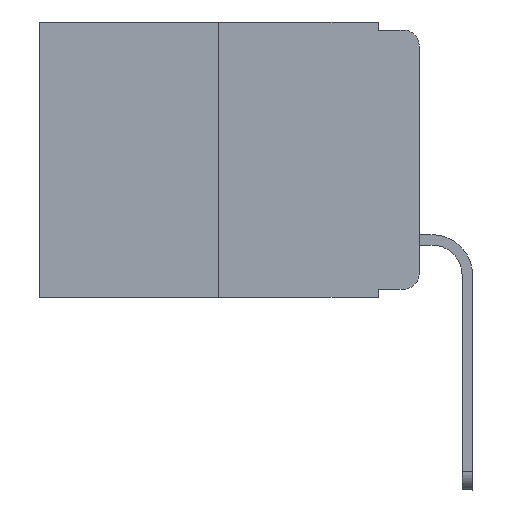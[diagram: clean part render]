
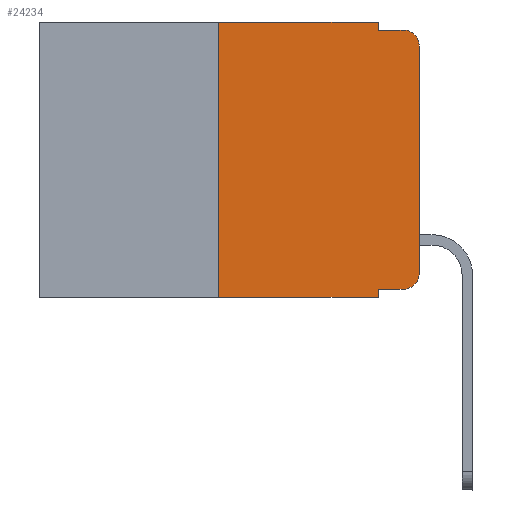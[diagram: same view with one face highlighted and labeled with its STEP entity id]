
A CAD part, left-side view. The second image highlights one B-rep face of the part: STEP entity #24234.
In plain terms, the highlighted planar face has unit normal (-1, 0, 0).
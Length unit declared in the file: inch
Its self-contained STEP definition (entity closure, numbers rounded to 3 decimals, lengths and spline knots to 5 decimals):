
#444 = DIRECTION ( 'NONE',  ( -1., 0., 0. ) ) ;
#1113 = VECTOR ( 'NONE', #25519, 39.37008 ) ;
#1357 = CARTESIAN_POINT ( 'NONE',  ( 0., 0., -0.313 ) ) ;
#1689 = VECTOR ( 'NONE', #13543, 39.37008 ) ;
#2533 = DIRECTION ( 'NONE',  ( 0., 0., -1. ) ) ;
#2951 = AXIS2_PLACEMENT_3D ( 'NONE', #6365, #25494, #16071 ) ;
#3312 = VERTEX_POINT ( 'NONE', #7951 ) ;
#3314 = EDGE_CURVE ( 'NONE', #19321, #23801, #14136, .T. ) ;
#3338 = PLANE ( 'NONE',  #13207 ) ;
#3358 = ORIENTED_EDGE ( 'NONE', *, *, #18865, .T. ) ;
#3513 = ORIENTED_EDGE ( 'NONE', *, *, #6354, .F. ) ;
#3849 = VERTEX_POINT ( 'NONE', #24023 ) ;
#4046 = LINE ( 'NONE', #19809, #18910 ) ;
#4088 = ORIENTED_EDGE ( 'NONE', *, *, #21610, .T. ) ;
#4286 = CARTESIAN_POINT ( 'NONE',  ( 0., 0., -0.03 ) ) ;
#4372 = EDGE_CURVE ( 'NONE', #3312, #18148, #19312, .T. ) ;
#4451 = VERTEX_POINT ( 'NONE', #1357 ) ;
#4537 = CARTESIAN_POINT ( 'NONE',  ( 0., 0.473, 0. ) ) ;
#5300 = DIRECTION ( 'NONE',  ( 1., 0., 0. ) ) ;
#5355 = CARTESIAN_POINT ( 'NONE',  ( 0., 0.051, -0.333 ) ) ;
#5700 = ORIENTED_EDGE ( 'NONE', *, *, #12153, .F. ) ;
#6138 = CARTESIAN_POINT ( 'NONE',  ( 0., 0.051, -0.01 ) ) ;
#6354 = EDGE_CURVE ( 'NONE', #18148, #3849, #22216, .T. ) ;
#6365 = CARTESIAN_POINT ( 'NONE',  ( 0., 0.02, -0.03 ) ) ;
#7677 = DIRECTION ( 'NONE',  ( 0., -1., 0. ) ) ;
#7944 = LINE ( 'NONE', #23806, #9525 ) ;
#7951 = CARTESIAN_POINT ( 'NONE',  ( 0., 0.25, -0.343 ) ) ;
#8575 = DIRECTION ( 'NONE',  ( 0., -1., 0. ) ) ;
#8639 = CARTESIAN_POINT ( 'NONE',  ( 0., 0.051, 0. ) ) ;
#9076 = ORIENTED_EDGE ( 'NONE', *, *, #4372, .F. ) ;
#9525 = VECTOR ( 'NONE', #15823, 39.37008 ) ;
#9788 = VECTOR ( 'NONE', #2533, 39.37008 ) ;
#11588 = EDGE_CURVE ( 'NONE', #3312, #15879, #23424, .T. ) ;
#12124 = CARTESIAN_POINT ( 'NONE',  ( 0., 0.25, 0. ) ) ;
#12153 = EDGE_CURVE ( 'NONE', #3849, #19693, #18287, .T. ) ;
#12673 = EDGE_CURVE ( 'NONE', #21593, #4451, #22116, .T. ) ;
#13207 = AXIS2_PLACEMENT_3D ( 'NONE', #22996, #5300, #13209 ) ;
#13209 = DIRECTION ( 'NONE',  ( 0., 0., -1. ) ) ;
#13543 = DIRECTION ( 'NONE',  ( 0., 0., 1. ) ) ;
#13728 = ORIENTED_EDGE ( 'NONE', *, *, #11588, .T. ) ;
#13797 = VERTEX_POINT ( 'NONE', #19602 ) ;
#14136 = CIRCLE ( 'NONE', #2951, 0.02 ) ;
#14393 = EDGE_LOOP ( 'NONE', ( #4088, #25323, #18531, #5700, #3513, #9076, #13728, #20049, #3358, #18759 ) ) ;
#14512 = VECTOR ( 'NONE', #8575, 39.37008 ) ;
#15823 = DIRECTION ( 'NONE',  ( 0., 0., -1. ) ) ;
#15879 = VERTEX_POINT ( 'NONE', #25448 ) ;
#16071 = DIRECTION ( 'NONE',  ( 0., 0., -1. ) ) ;
#17545 = VECTOR ( 'NONE', #7677, 39.37008 ) ;
#17872 = CARTESIAN_POINT ( 'NONE',  ( 0., 0.02, -0.333 ) ) ;
#18023 = AXIS2_PLACEMENT_3D ( 'NONE', #20078, #444, #18518 ) ;
#18148 = VERTEX_POINT ( 'NONE', #12124 ) ;
#18287 = LINE ( 'NONE', #8639, #9788 ) ;
#18518 = DIRECTION ( 'NONE',  ( 0., 0., -1. ) ) ;
#18531 = ORIENTED_EDGE ( 'NONE', *, *, #20002, .F. ) ;
#18649 = DIRECTION ( 'NONE',  ( 0., -1., 0. ) ) ;
#18759 = ORIENTED_EDGE ( 'NONE', *, *, #12673, .T. ) ;
#18865 = EDGE_CURVE ( 'NONE', #13797, #21593, #23177, .T. ) ;
#18910 = VECTOR ( 'NONE', #19933, 39.37008 ) ;
#18985 = FACE_OUTER_BOUND ( 'NONE', #14393, .T. ) ;
#19312 = LINE ( 'NONE', #21107, #1689 ) ;
#19321 = VERTEX_POINT ( 'NONE', #4286 ) ;
#19602 = CARTESIAN_POINT ( 'NONE',  ( 0., 0.051, -0.333 ) ) ;
#19693 = VERTEX_POINT ( 'NONE', #20369 ) ;
#19809 = CARTESIAN_POINT ( 'NONE',  ( 0., 0., 0. ) ) ;
#19933 = DIRECTION ( 'NONE',  ( 0., 0., 1. ) ) ;
#20002 = EDGE_CURVE ( 'NONE', #19693, #23801, #21389, .T. ) ;
#20049 = ORIENTED_EDGE ( 'NONE', *, *, #23575, .F. ) ;
#20078 = CARTESIAN_POINT ( 'NONE',  ( 0., 0.02, -0.313 ) ) ;
#20369 = CARTESIAN_POINT ( 'NONE',  ( 0., 0.051, -0.01 ) ) ;
#21107 = CARTESIAN_POINT ( 'NONE',  ( 0., 0.25, 0. ) ) ;
#21389 = LINE ( 'NONE', #6138, #1113 ) ;
#21593 = VERTEX_POINT ( 'NONE', #17872 ) ;
#21610 = EDGE_CURVE ( 'NONE', #4451, #19321, #4046, .T. ) ;
#22116 = CIRCLE ( 'NONE', #18023, 0.02 ) ;
#22216 = LINE ( 'NONE', #4537, #14512 ) ;
#22996 = CARTESIAN_POINT ( 'NONE',  ( 0., 0.473, 0. ) ) ;
#23177 = LINE ( 'NONE', #5355, #23735 ) ;
#23424 = LINE ( 'NONE', #25474, #17545 ) ;
#23575 = EDGE_CURVE ( 'NONE', #13797, #15879, #7944, .T. ) ;
#23735 = VECTOR ( 'NONE', #18649, 39.37008 ) ;
#23801 = VERTEX_POINT ( 'NONE', #24950 ) ;
#23806 = CARTESIAN_POINT ( 'NONE',  ( 0., 0.051, 0. ) ) ;
#24023 = CARTESIAN_POINT ( 'NONE',  ( 0., 0.051, 0. ) ) ;
#24234 = ADVANCED_FACE ( 'NONE', ( #18985 ), #3338, .F. ) ;
#24950 = CARTESIAN_POINT ( 'NONE',  ( 0., 0.02, -0.01 ) ) ;
#25323 = ORIENTED_EDGE ( 'NONE', *, *, #3314, .T. ) ;
#25448 = CARTESIAN_POINT ( 'NONE',  ( 0., 0.051, -0.343 ) ) ;
#25474 = CARTESIAN_POINT ( 'NONE',  ( 0., 0.473, -0.343 ) ) ;
#25494 = DIRECTION ( 'NONE',  ( -1., 0., 0. ) ) ;
#25519 = DIRECTION ( 'NONE',  ( 0., -1., 0. ) ) ;
